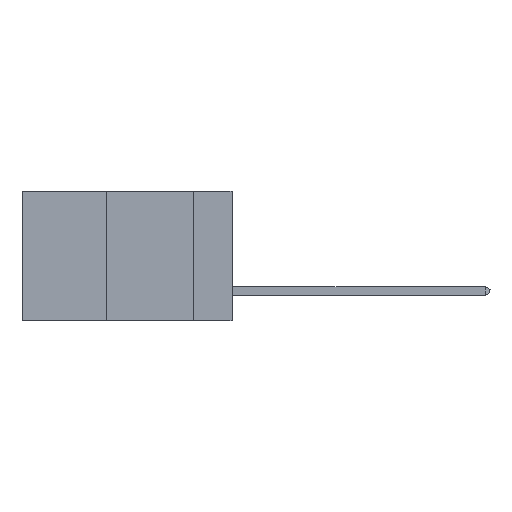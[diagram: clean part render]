
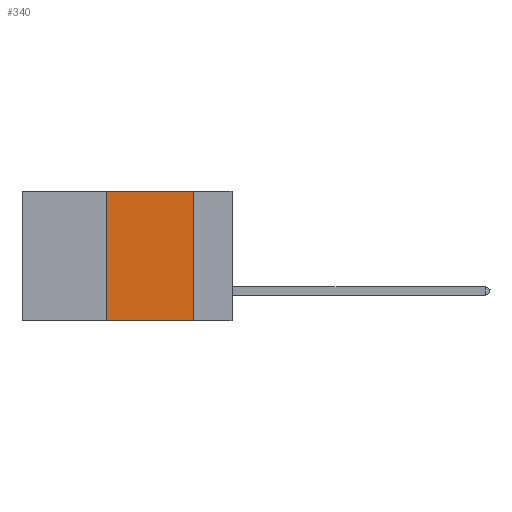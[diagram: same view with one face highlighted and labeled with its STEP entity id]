
A CAD part, left-side view. The second image highlights one B-rep face of the part: STEP entity #340.
In plain terms, the highlighted planar face has unit normal (-1, 0, 0).
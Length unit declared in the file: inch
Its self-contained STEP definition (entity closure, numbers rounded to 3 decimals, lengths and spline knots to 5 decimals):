
#340 = ADVANCED_FACE ( 'NONE', ( #17549 ), #5055, .F. ) ;
#485 = DIRECTION ( 'NONE',  ( 0., 0., -1. ) ) ;
#1291 = VECTOR ( 'NONE', #1574, 39.37008 ) ;
#1574 = DIRECTION ( 'NONE',  ( 0., 0., 1. ) ) ;
#1741 = EDGE_CURVE ( 'NONE', #14880, #10194, #16939, .T. ) ;
#3330 = ORIENTED_EDGE ( 'NONE', *, *, #12348, .F. ) ;
#3703 = CARTESIAN_POINT ( 'NONE',  ( 0., 0.36, 0. ) ) ;
#4251 = CARTESIAN_POINT ( 'NONE',  ( 0., 0.11, 0. ) ) ;
#4694 = CARTESIAN_POINT ( 'NONE',  ( 0., 0.6, 0. ) ) ;
#4735 = ORIENTED_EDGE ( 'NONE', *, *, #14045, .T. ) ;
#5055 = PLANE ( 'NONE',  #11823 ) ;
#5416 = LINE ( 'NONE', #19136, #1291 ) ;
#6416 = VECTOR ( 'NONE', #16320, 39.37008 ) ;
#6694 = LINE ( 'NONE', #4694, #6416 ) ;
#7082 = CARTESIAN_POINT ( 'NONE',  ( 0., 0.11, -0.37 ) ) ;
#7178 = VECTOR ( 'NONE', #20506, 39.37008 ) ;
#7311 = CARTESIAN_POINT ( 'NONE',  ( 0., 0.36, -0.37 ) ) ;
#8307 = CARTESIAN_POINT ( 'NONE',  ( 0., 0.6, 0. ) ) ;
#9663 = ORIENTED_EDGE ( 'NONE', *, *, #13377, .F. ) ;
#9697 = EDGE_LOOP ( 'NONE', ( #16246, #3330, #9663, #4735 ) ) ;
#9995 = DIRECTION ( 'NONE',  ( 1., 0., 0. ) ) ;
#10194 = VERTEX_POINT ( 'NONE', #7082 ) ;
#11751 = DIRECTION ( 'NONE',  ( 0., 0., -1. ) ) ;
#11823 = AXIS2_PLACEMENT_3D ( 'NONE', #8307, #9995, #11751 ) ;
#12348 = EDGE_CURVE ( 'NONE', #15255, #14880, #6694, .T. ) ;
#13377 = EDGE_CURVE ( 'NONE', #15679, #15255, #5416, .T. ) ;
#14045 = EDGE_CURVE ( 'NONE', #15679, #10194, #20846, .T. ) ;
#14880 = VERTEX_POINT ( 'NONE', #4251 ) ;
#15255 = VERTEX_POINT ( 'NONE', #3703 ) ;
#15393 = CARTESIAN_POINT ( 'NONE',  ( 0., 0.6, -0.37 ) ) ;
#15679 = VERTEX_POINT ( 'NONE', #7311 ) ;
#16246 = ORIENTED_EDGE ( 'NONE', *, *, #1741, .F. ) ;
#16320 = DIRECTION ( 'NONE',  ( 0., -1., 0. ) ) ;
#16939 = LINE ( 'NONE', #18345, #20496 ) ;
#17549 = FACE_OUTER_BOUND ( 'NONE', #9697, .T. ) ;
#18345 = CARTESIAN_POINT ( 'NONE',  ( 0., 0.11, 0. ) ) ;
#19136 = CARTESIAN_POINT ( 'NONE',  ( 0., 0.36, 0. ) ) ;
#20496 = VECTOR ( 'NONE', #485, 39.37008 ) ;
#20506 = DIRECTION ( 'NONE',  ( 0., -1., 0. ) ) ;
#20846 = LINE ( 'NONE', #15393, #7178 ) ;
